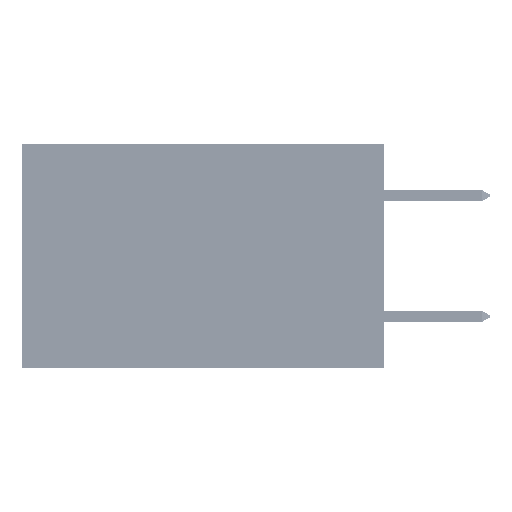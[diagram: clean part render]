
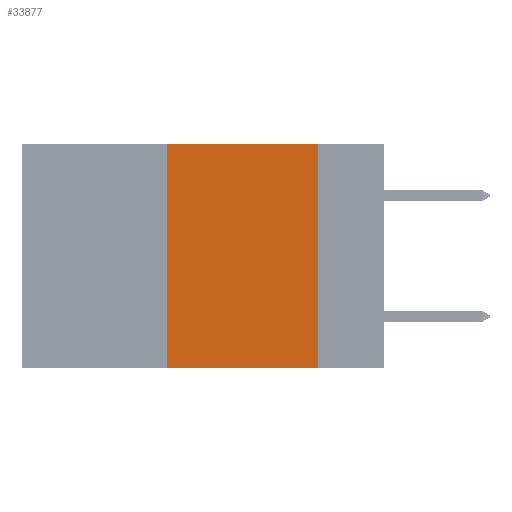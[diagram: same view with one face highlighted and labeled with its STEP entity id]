
A CAD part, left-side view. The second image highlights one B-rep face of the part: STEP entity #33877.
In plain terms, the highlighted planar face has unit normal (-1, 0, 0).
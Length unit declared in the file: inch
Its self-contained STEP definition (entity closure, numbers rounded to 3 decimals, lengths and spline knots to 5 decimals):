
#692 = ORIENTED_EDGE ( 'NONE', *, *, #46083, .F. ) ;
#1569 = CARTESIAN_POINT ( 'NONE',  ( 0., 0.6, 0. ) ) ;
#3978 = ORIENTED_EDGE ( 'NONE', *, *, #32362, .F. ) ;
#8782 = DIRECTION ( 'NONE',  ( 0., 0., 1. ) ) ;
#11336 = CARTESIAN_POINT ( 'NONE',  ( 0., 0.6, -0.37 ) ) ;
#13276 = VECTOR ( 'NONE', #8782, 39.37008 ) ;
#13875 = PLANE ( 'NONE',  #19366 ) ;
#15075 = EDGE_CURVE ( 'NONE', #37837, #31954, #20241, .T. ) ;
#17913 = FACE_OUTER_BOUND ( 'NONE', #46236, .T. ) ;
#19366 = AXIS2_PLACEMENT_3D ( 'NONE', #21509, #39950, #46435 ) ;
#20237 = DIRECTION ( 'NONE',  ( 0., 0., -1. ) ) ;
#20241 = LINE ( 'NONE', #1569, #24336 ) ;
#21509 = CARTESIAN_POINT ( 'NONE',  ( 0., 0.6, 0. ) ) ;
#23292 = CARTESIAN_POINT ( 'NONE',  ( 0., 0.11, -0.37 ) ) ;
#23502 = DIRECTION ( 'NONE',  ( 0., -1., 0. ) ) ;
#23662 = VERTEX_POINT ( 'NONE', #23292 ) ;
#24336 = VECTOR ( 'NONE', #41811, 39.37008 ) ;
#25375 = VECTOR ( 'NONE', #20237, 39.37008 ) ;
#26656 = ORIENTED_EDGE ( 'NONE', *, *, #35057, .T. ) ;
#27218 = LINE ( 'NONE', #34408, #13276 ) ;
#27678 = CARTESIAN_POINT ( 'NONE',  ( 0., 0.11, 0. ) ) ;
#29033 = VERTEX_POINT ( 'NONE', #44429 ) ;
#31132 = CARTESIAN_POINT ( 'NONE',  ( 0., 0.11, 0. ) ) ;
#31194 = CARTESIAN_POINT ( 'NONE',  ( 0., 0.36, 0. ) ) ;
#31954 = VERTEX_POINT ( 'NONE', #31132 ) ;
#32362 = EDGE_CURVE ( 'NONE', #31954, #23662, #35101, .T. ) ;
#33877 = ADVANCED_FACE ( 'NONE', ( #17913 ), #13875, .F. ) ;
#34408 = CARTESIAN_POINT ( 'NONE',  ( 0., 0.36, 0. ) ) ;
#35057 = EDGE_CURVE ( 'NONE', #29033, #23662, #44150, .T. ) ;
#35101 = LINE ( 'NONE', #27678, #25375 ) ;
#37837 = VERTEX_POINT ( 'NONE', #31194 ) ;
#39950 = DIRECTION ( 'NONE',  ( 1., 0., 0. ) ) ;
#41627 = VECTOR ( 'NONE', #23502, 39.37008 ) ;
#41811 = DIRECTION ( 'NONE',  ( 0., -1., 0. ) ) ;
#44150 = LINE ( 'NONE', #11336, #41627 ) ;
#44429 = CARTESIAN_POINT ( 'NONE',  ( 0., 0.36, -0.37 ) ) ;
#46083 = EDGE_CURVE ( 'NONE', #29033, #37837, #27218, .T. ) ;
#46236 = EDGE_LOOP ( 'NONE', ( #3978, #46485, #692, #26656 ) ) ;
#46435 = DIRECTION ( 'NONE',  ( 0., 0., -1. ) ) ;
#46485 = ORIENTED_EDGE ( 'NONE', *, *, #15075, .F. ) ;
